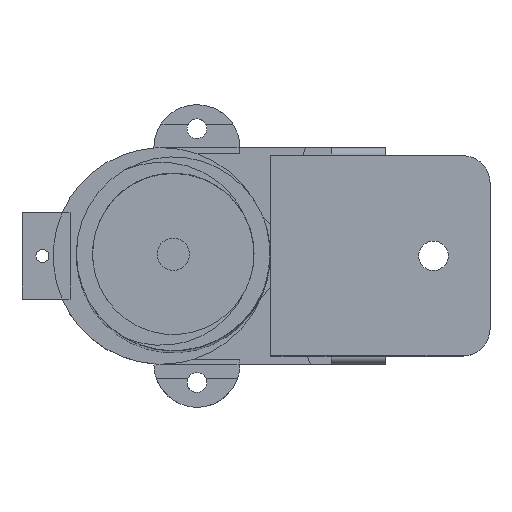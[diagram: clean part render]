
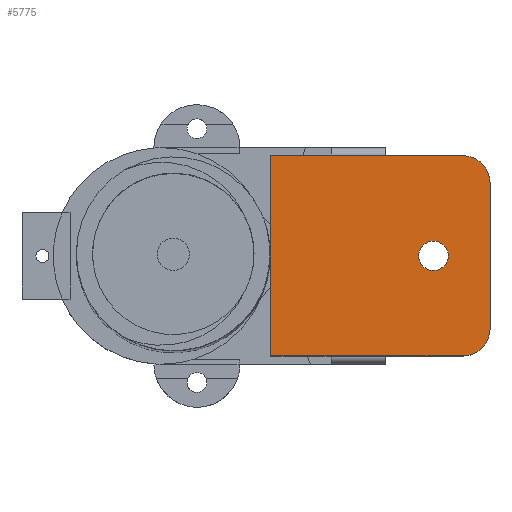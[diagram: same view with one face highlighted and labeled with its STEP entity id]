
A CAD part, top view. The second image highlights one B-rep face of the part: STEP entity #5775.
In plain terms, the highlighted planar face has unit normal (0, 0, 1).
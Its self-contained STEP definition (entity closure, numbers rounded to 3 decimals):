
#3618 = PLANE('',#3619);
#3619 = AXIS2_PLACEMENT_3D('',#3620,#3621,#3622);
#3620 = CARTESIAN_POINT('',(-27.612,18.6,22.6));
#3621 = DIRECTION('',(0.,1.,0.));
#3622 = DIRECTION('',(1.,0.,0.));
#4226 = PLANE('',#4227);
#4227 = AXIS2_PLACEMENT_3D('',#4228,#4229,#4230);
#4228 = CARTESIAN_POINT('',(13.137,-18.6,22.6));
#4229 = DIRECTION('',(0.,-1.,0.));
#4230 = DIRECTION('',(-1.,0.,0.));
#4845 = PLANE('',#4846);
#4846 = AXIS2_PLACEMENT_3D('',#4847,#4848,#4849);
#4847 = CARTESIAN_POINT('',(-27.612,-18.6,22.6));
#4848 = DIRECTION('',(-1.,0.,0.));
#4849 = DIRECTION('',(0.,1.,0.));
#4882 = EDGE_CURVE('',#4883,#4885,#4887,.T.);
#4883 = VERTEX_POINT('',#4884);
#4884 = CARTESIAN_POINT('',(-27.612,18.6,24.1));
#4885 = VERTEX_POINT('',#4886);
#4886 = CARTESIAN_POINT('',(8.137,18.6,24.1));
#4887 = SURFACE_CURVE('',#4888,(#4892,#4899),.PCURVE_S1.);
#4888 = LINE('',#4889,#4890);
#4889 = CARTESIAN_POINT('',(-27.612,18.6,24.1));
#4890 = VECTOR('',#4891,1.);
#4891 = DIRECTION('',(1.,0.,0.));
#4892 = PCURVE('',#3618,#4893);
#4893 = DEFINITIONAL_REPRESENTATION('',(#4894),#4898);
#4894 = LINE('',#4895,#4896);
#4895 = CARTESIAN_POINT('',(0.,-1.5));
#4896 = VECTOR('',#4897,1.);
#4897 = DIRECTION('',(1.,0.));
#4898 = ( GEOMETRIC_REPRESENTATION_CONTEXT(2) 
PARAMETRIC_REPRESENTATION_CONTEXT() REPRESENTATION_CONTEXT('2D SPACE',''
  ) );
#4899 = PCURVE('',#4900,#4905);
#4900 = PLANE('',#4901);
#4901 = AXIS2_PLACEMENT_3D('',#4902,#4903,#4904);
#4902 = CARTESIAN_POINT('',(-27.612,18.6,24.1));
#4903 = DIRECTION('',(0.,0.,1.));
#4904 = DIRECTION('',(1.,0.,0.));
#4905 = DEFINITIONAL_REPRESENTATION('',(#4906),#4910);
#4906 = LINE('',#4907,#4908);
#4907 = CARTESIAN_POINT('',(0.,0.));
#4908 = VECTOR('',#4909,1.);
#4909 = DIRECTION('',(1.,0.));
#4910 = ( GEOMETRIC_REPRESENTATION_CONTEXT(2) 
PARAMETRIC_REPRESENTATION_CONTEXT() REPRESENTATION_CONTEXT('2D SPACE',''
  ) );
#4928 = CYLINDRICAL_SURFACE('',#4929,5.);
#4929 = AXIS2_PLACEMENT_3D('',#4930,#4931,#4932);
#4930 = CARTESIAN_POINT('',(8.137,13.6,22.6));
#4931 = DIRECTION('',(0.,0.,1.));
#4932 = DIRECTION('',(1.,0.,0.));
#5292 = EDGE_CURVE('',#5293,#5295,#5297,.T.);
#5293 = VERTEX_POINT('',#5294);
#5294 = CARTESIAN_POINT('',(8.137,-18.6,24.1));
#5295 = VERTEX_POINT('',#5296);
#5296 = CARTESIAN_POINT('',(-27.612,-18.6,24.1));
#5297 = SURFACE_CURVE('',#5298,(#5302,#5309),.PCURVE_S1.);
#5298 = LINE('',#5299,#5300);
#5299 = CARTESIAN_POINT('',(13.137,-18.6,24.1));
#5300 = VECTOR('',#5301,1.);
#5301 = DIRECTION('',(-1.,0.,0.));
#5302 = PCURVE('',#4226,#5303);
#5303 = DEFINITIONAL_REPRESENTATION('',(#5304),#5308);
#5304 = LINE('',#5305,#5306);
#5305 = CARTESIAN_POINT('',(0.,-1.5));
#5306 = VECTOR('',#5307,1.);
#5307 = DIRECTION('',(1.,0.));
#5308 = ( GEOMETRIC_REPRESENTATION_CONTEXT(2) 
PARAMETRIC_REPRESENTATION_CONTEXT() REPRESENTATION_CONTEXT('2D SPACE',''
  ) );
#5309 = PCURVE('',#4900,#5310);
#5310 = DEFINITIONAL_REPRESENTATION('',(#5311),#5315);
#5311 = LINE('',#5312,#5313);
#5312 = CARTESIAN_POINT('',(40.749,-37.2));
#5313 = VECTOR('',#5314,1.);
#5314 = DIRECTION('',(-1.,0.));
#5315 = ( GEOMETRIC_REPRESENTATION_CONTEXT(2) 
PARAMETRIC_REPRESENTATION_CONTEXT() REPRESENTATION_CONTEXT('2D SPACE',''
  ) );
#5356 = CYLINDRICAL_SURFACE('',#5357,5.);
#5357 = AXIS2_PLACEMENT_3D('',#5358,#5359,#5360);
#5358 = CARTESIAN_POINT('',(8.137,-13.6,22.6));
#5359 = DIRECTION('',(0.,0.,1.));
#5360 = DIRECTION('',(1.,0.,0.));
#5753 = EDGE_CURVE('',#5295,#4883,#5754,.T.);
#5754 = SURFACE_CURVE('',#5755,(#5759,#5766),.PCURVE_S1.);
#5755 = LINE('',#5756,#5757);
#5756 = CARTESIAN_POINT('',(-27.612,-18.6,24.1));
#5757 = VECTOR('',#5758,1.);
#5758 = DIRECTION('',(0.,1.,0.));
#5759 = PCURVE('',#4845,#5760);
#5760 = DEFINITIONAL_REPRESENTATION('',(#5761),#5765);
#5761 = LINE('',#5762,#5763);
#5762 = CARTESIAN_POINT('',(0.,-1.5));
#5763 = VECTOR('',#5764,1.);
#5764 = DIRECTION('',(1.,0.));
#5765 = ( GEOMETRIC_REPRESENTATION_CONTEXT(2) 
PARAMETRIC_REPRESENTATION_CONTEXT() REPRESENTATION_CONTEXT('2D SPACE',''
  ) );
#5766 = PCURVE('',#4900,#5767);
#5767 = DEFINITIONAL_REPRESENTATION('',(#5768),#5772);
#5768 = LINE('',#5769,#5770);
#5769 = CARTESIAN_POINT('',(0.,-37.2));
#5770 = VECTOR('',#5771,1.);
#5771 = DIRECTION('',(0.,1.));
#5772 = ( GEOMETRIC_REPRESENTATION_CONTEXT(2) 
PARAMETRIC_REPRESENTATION_CONTEXT() REPRESENTATION_CONTEXT('2D SPACE',''
  ) );
#5775 = ADVANCED_FACE('',(#5776,#5859),#4900,.T.);
#5776 = FACE_BOUND('',#5777,.T.);
#5777 = EDGE_LOOP('',(#5778,#5808,#5830,#5831,#5832,#5833));
#5778 = ORIENTED_EDGE('',*,*,#5779,.F.);
#5779 = EDGE_CURVE('',#5780,#5782,#5784,.T.);
#5780 = VERTEX_POINT('',#5781);
#5781 = CARTESIAN_POINT('',(13.137,13.6,24.1));
#5782 = VERTEX_POINT('',#5783);
#5783 = CARTESIAN_POINT('',(13.137,-13.6,24.1));
#5784 = SURFACE_CURVE('',#5785,(#5789,#5796),.PCURVE_S1.);
#5785 = LINE('',#5786,#5787);
#5786 = CARTESIAN_POINT('',(13.137,18.6,24.1));
#5787 = VECTOR('',#5788,1.);
#5788 = DIRECTION('',(0.,-1.,0.));
#5789 = PCURVE('',#4900,#5790);
#5790 = DEFINITIONAL_REPRESENTATION('',(#5791),#5795);
#5791 = LINE('',#5792,#5793);
#5792 = CARTESIAN_POINT('',(40.749,0.));
#5793 = VECTOR('',#5794,1.);
#5794 = DIRECTION('',(0.,-1.));
#5795 = ( GEOMETRIC_REPRESENTATION_CONTEXT(2) 
PARAMETRIC_REPRESENTATION_CONTEXT() REPRESENTATION_CONTEXT('2D SPACE',''
  ) );
#5796 = PCURVE('',#5797,#5802);
#5797 = PLANE('',#5798);
#5798 = AXIS2_PLACEMENT_3D('',#5799,#5800,#5801);
#5799 = CARTESIAN_POINT('',(13.137,18.6,22.6));
#5800 = DIRECTION('',(1.,0.,0.));
#5801 = DIRECTION('',(0.,-1.,0.));
#5802 = DEFINITIONAL_REPRESENTATION('',(#5803),#5807);
#5803 = LINE('',#5804,#5805);
#5804 = CARTESIAN_POINT('',(0.,-1.5));
#5805 = VECTOR('',#5806,1.);
#5806 = DIRECTION('',(1.,0.));
#5807 = ( GEOMETRIC_REPRESENTATION_CONTEXT(2) 
PARAMETRIC_REPRESENTATION_CONTEXT() REPRESENTATION_CONTEXT('2D SPACE',''
  ) );
#5808 = ORIENTED_EDGE('',*,*,#5809,.T.);
#5809 = EDGE_CURVE('',#5780,#4885,#5810,.T.);
#5810 = SURFACE_CURVE('',#5811,(#5816,#5823),.PCURVE_S1.);
#5811 = CIRCLE('',#5812,5.);
#5812 = AXIS2_PLACEMENT_3D('',#5813,#5814,#5815);
#5813 = CARTESIAN_POINT('',(8.137,13.6,24.1));
#5814 = DIRECTION('',(0.,0.,1.));
#5815 = DIRECTION('',(0.,-1.,0.));
#5816 = PCURVE('',#4900,#5817);
#5817 = DEFINITIONAL_REPRESENTATION('',(#5818),#5822);
#5818 = CIRCLE('',#5819,5.);
#5819 = AXIS2_PLACEMENT_2D('',#5820,#5821);
#5820 = CARTESIAN_POINT('',(35.749,-5.));
#5821 = DIRECTION('',(0.,-1.));
#5822 = ( GEOMETRIC_REPRESENTATION_CONTEXT(2) 
PARAMETRIC_REPRESENTATION_CONTEXT() REPRESENTATION_CONTEXT('2D SPACE',''
  ) );
#5823 = PCURVE('',#4928,#5824);
#5824 = DEFINITIONAL_REPRESENTATION('',(#5825),#5829);
#5825 = LINE('',#5826,#5827);
#5826 = CARTESIAN_POINT('',(-1.571,1.5));
#5827 = VECTOR('',#5828,1.);
#5828 = DIRECTION('',(1.,0.));
#5829 = ( GEOMETRIC_REPRESENTATION_CONTEXT(2) 
PARAMETRIC_REPRESENTATION_CONTEXT() REPRESENTATION_CONTEXT('2D SPACE',''
  ) );
#5830 = ORIENTED_EDGE('',*,*,#4882,.F.);
#5831 = ORIENTED_EDGE('',*,*,#5753,.F.);
#5832 = ORIENTED_EDGE('',*,*,#5292,.F.);
#5833 = ORIENTED_EDGE('',*,*,#5834,.F.);
#5834 = EDGE_CURVE('',#5782,#5293,#5835,.T.);
#5835 = SURFACE_CURVE('',#5836,(#5841,#5852),.PCURVE_S1.);
#5836 = CIRCLE('',#5837,5.);
#5837 = AXIS2_PLACEMENT_3D('',#5838,#5839,#5840);
#5838 = CARTESIAN_POINT('',(8.137,-13.6,24.1));
#5839 = DIRECTION('',(0.,0.,-1.));
#5840 = DIRECTION('',(0.,-1.,0.));
#5841 = PCURVE('',#4900,#5842);
#5842 = DEFINITIONAL_REPRESENTATION('',(#5843),#5851);
#5843 = ( BOUNDED_CURVE() B_SPLINE_CURVE(2,(#5844,#5845,#5846,#5847,
#5848,#5849,#5850),.UNSPECIFIED.,.T.,.F.) B_SPLINE_CURVE_WITH_KNOTS((1,2
    ,2,2,2,1),(-2.094,0.,2.094,4.189,
6.283,8.378),.UNSPECIFIED.) CURVE() 
GEOMETRIC_REPRESENTATION_ITEM() RATIONAL_B_SPLINE_CURVE((1.,0.5,1.,0.5,
1.,0.5,1.)) REPRESENTATION_ITEM('') );
#5844 = CARTESIAN_POINT('',(35.749,-37.2));
#5845 = CARTESIAN_POINT('',(27.089,-37.2));
#5846 = CARTESIAN_POINT('',(31.419,-29.7));
#5847 = CARTESIAN_POINT('',(35.749,-22.2));
#5848 = CARTESIAN_POINT('',(40.079,-29.7));
#5849 = CARTESIAN_POINT('',(44.409,-37.2));
#5850 = CARTESIAN_POINT('',(35.749,-37.2));
#5851 = ( GEOMETRIC_REPRESENTATION_CONTEXT(2) 
PARAMETRIC_REPRESENTATION_CONTEXT() REPRESENTATION_CONTEXT('2D SPACE',''
  ) );
#5852 = PCURVE('',#5356,#5853);
#5853 = DEFINITIONAL_REPRESENTATION('',(#5854),#5858);
#5854 = LINE('',#5855,#5856);
#5855 = CARTESIAN_POINT('',(4.712,1.5));
#5856 = VECTOR('',#5857,1.);
#5857 = DIRECTION('',(-1.,0.));
#5858 = ( GEOMETRIC_REPRESENTATION_CONTEXT(2) 
PARAMETRIC_REPRESENTATION_CONTEXT() REPRESENTATION_CONTEXT('2D SPACE',''
  ) );
#5859 = FACE_BOUND('',#5860,.T.);
#5860 = EDGE_LOOP('',(#5861));
#5861 = ORIENTED_EDGE('',*,*,#5862,.T.);
#5862 = EDGE_CURVE('',#5863,#5863,#5865,.T.);
#5863 = VERTEX_POINT('',#5864);
#5864 = CARTESIAN_POINT('',(5.387,0.,24.1));
#5865 = SURFACE_CURVE('',#5866,(#5871,#5882),.PCURVE_S1.);
#5866 = CIRCLE('',#5867,2.75);
#5867 = AXIS2_PLACEMENT_3D('',#5868,#5869,#5870);
#5868 = CARTESIAN_POINT('',(2.637,0.,24.1));
#5869 = DIRECTION('',(0.,0.,-1.));
#5870 = DIRECTION('',(1.,0.,0.));
#5871 = PCURVE('',#4900,#5872);
#5872 = DEFINITIONAL_REPRESENTATION('',(#5873),#5881);
#5873 = ( BOUNDED_CURVE() B_SPLINE_CURVE(2,(#5874,#5875,#5876,#5877,
#5878,#5879,#5880),.UNSPECIFIED.,.F.,.F.) B_SPLINE_CURVE_WITH_KNOTS((1,2
    ,2,2,2,1),(-2.094,0.,2.094,4.189,
6.283,8.378),.UNSPECIFIED.) CURVE() 
GEOMETRIC_REPRESENTATION_ITEM() RATIONAL_B_SPLINE_CURVE((1.,0.5,1.,0.5,
1.,0.5,1.)) REPRESENTATION_ITEM('') );
#5874 = CARTESIAN_POINT('',(32.999,-18.6));
#5875 = CARTESIAN_POINT('',(32.999,-23.363));
#5876 = CARTESIAN_POINT('',(28.874,-20.982));
#5877 = CARTESIAN_POINT('',(24.749,-18.6));
#5878 = CARTESIAN_POINT('',(28.874,-16.218));
#5879 = CARTESIAN_POINT('',(32.999,-13.837));
#5880 = CARTESIAN_POINT('',(32.999,-18.6));
#5881 = ( GEOMETRIC_REPRESENTATION_CONTEXT(2) 
PARAMETRIC_REPRESENTATION_CONTEXT() REPRESENTATION_CONTEXT('2D SPACE',''
  ) );
#5882 = PCURVE('',#5883,#5888);
#5883 = CYLINDRICAL_SURFACE('',#5884,2.75);
#5884 = AXIS2_PLACEMENT_3D('',#5885,#5886,#5887);
#5885 = CARTESIAN_POINT('',(2.637,0.,0.));
#5886 = DIRECTION('',(0.,0.,-1.));
#5887 = DIRECTION('',(1.,0.,0.));
#5888 = DEFINITIONAL_REPRESENTATION('',(#5889),#5893);
#5889 = LINE('',#5890,#5891);
#5890 = CARTESIAN_POINT('',(0.,-24.1));
#5891 = VECTOR('',#5892,1.);
#5892 = DIRECTION('',(1.,0.));
#5893 = ( GEOMETRIC_REPRESENTATION_CONTEXT(2) 
PARAMETRIC_REPRESENTATION_CONTEXT() REPRESENTATION_CONTEXT('2D SPACE',''
  ) );
